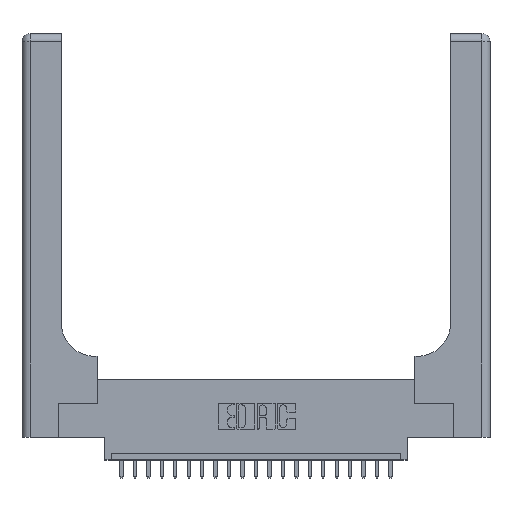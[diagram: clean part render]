
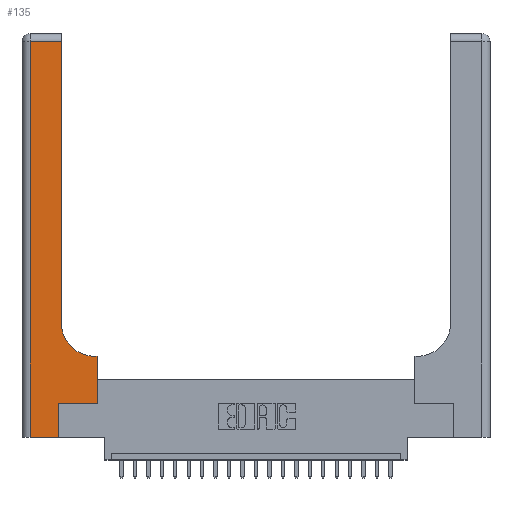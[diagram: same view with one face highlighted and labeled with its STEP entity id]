
A CAD part, top view. The second image highlights one B-rep face of the part: STEP entity #135.
In plain terms, the highlighted planar face has unit normal (0, 0, 1).
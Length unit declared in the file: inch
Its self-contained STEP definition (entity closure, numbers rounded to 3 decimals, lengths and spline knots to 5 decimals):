
#114 = DIRECTION ( 'NONE',  ( 0., 1., 0. ) ) ;
#135 = ADVANCED_FACE ( 'NONE', ( #22724 ), #13976, .F. ) ;
#378 = CARTESIAN_POINT ( 'NONE',  ( 0., 2.94, 0.37 ) ) ;
#489 = VERTEX_POINT ( 'NONE', #5248 ) ;
#940 = CARTESIAN_POINT ( 'NONE',  ( 0., 0., 0.37 ) ) ;
#1065 = CARTESIAN_POINT ( 'NONE',  ( 0.06, 0., 0.37 ) ) ;
#1254 = ORIENTED_EDGE ( 'NONE', *, *, #21619, .T. ) ;
#1466 = DIRECTION ( 'NONE',  ( 0., -1., 0. ) ) ;
#1485 = DIRECTION ( 'NONE',  ( 0., 0., -1. ) ) ;
#1964 = CARTESIAN_POINT ( 'NONE',  ( 0.06, 2.94, 0.37 ) ) ;
#2144 = VERTEX_POINT ( 'NONE', #1065 ) ;
#2228 = CARTESIAN_POINT ( 'NONE',  ( 0.2915, 0.85, 0.37 ) ) ;
#2350 = VERTEX_POINT ( 'NONE', #19064 ) ;
#2406 = VECTOR ( 'NONE', #114, 39.37008 ) ;
#2436 = DIRECTION ( 'NONE',  ( 1., 0., 0. ) ) ;
#3029 = ORIENTED_EDGE ( 'NONE', *, *, #9383, .T. ) ;
#3120 = DIRECTION ( 'NONE',  ( 0., 1., 0. ) ) ;
#3335 = CARTESIAN_POINT ( 'NONE',  ( 0.5585, 0.25, 0.37 ) ) ;
#3462 = DIRECTION ( 'NONE',  ( 1., 0., 0. ) ) ;
#3573 = VERTEX_POINT ( 'NONE', #10100 ) ;
#3940 = EDGE_CURVE ( 'NONE', #23314, #2350, #17801, .T. ) ;
#5221 = VECTOR ( 'NONE', #14301, 39.37008 ) ;
#5248 = CARTESIAN_POINT ( 'NONE',  ( 0.269, 0., 0.37 ) ) ;
#6643 = ORIENTED_EDGE ( 'NONE', *, *, #7763, .T. ) ;
#6750 = VERTEX_POINT ( 'NONE', #1964 ) ;
#7763 = EDGE_CURVE ( 'NONE', #6750, #2144, #15623, .T. ) ;
#8022 = CIRCLE ( 'NONE', #17472, 0.25 ) ;
#8396 = DIRECTION ( 'NONE',  ( 1., 0., 0. ) ) ;
#8469 = VECTOR ( 'NONE', #9694, 39.37008 ) ;
#8691 = CARTESIAN_POINT ( 'NONE',  ( 0.269, 0.25, 0.37 ) ) ;
#8767 = CARTESIAN_POINT ( 'NONE',  ( 0.2915, 3., 0.37 ) ) ;
#8817 = EDGE_LOOP ( 'NONE', ( #12854, #9154, #6643, #3029, #10839, #1254, #19373, #16457, #23929 ) ) ;
#8840 = LINE ( 'NONE', #8767, #20716 ) ;
#8846 = DIRECTION ( 'NONE',  ( 0., 1., 0. ) ) ;
#9154 = ORIENTED_EDGE ( 'NONE', *, *, #10484, .T. ) ;
#9383 = EDGE_CURVE ( 'NONE', #2144, #489, #22143, .T. ) ;
#9637 = CARTESIAN_POINT ( 'NONE',  ( 0.269, 0.25, 0.37 ) ) ;
#9694 = DIRECTION ( 'NONE',  ( -1., 0., 0. ) ) ;
#10100 = CARTESIAN_POINT ( 'NONE',  ( 0.2915, 2.94, 0.37 ) ) ;
#10171 = LINE ( 'NONE', #18533, #5221 ) ;
#10422 = VERTEX_POINT ( 'NONE', #8691 ) ;
#10484 = EDGE_CURVE ( 'NONE', #3573, #6750, #21208, .T. ) ;
#10530 = CARTESIAN_POINT ( 'NONE',  ( 0.5415, 0.6, 0.37 ) ) ;
#10682 = VERTEX_POINT ( 'NONE', #2228 ) ;
#10839 = ORIENTED_EDGE ( 'NONE', *, *, #12359, .T. ) ;
#12359 = EDGE_CURVE ( 'NONE', #489, #10422, #13602, .T. ) ;
#12829 = AXIS2_PLACEMENT_3D ( 'NONE', #23503, #1485, #14568 ) ;
#12854 = ORIENTED_EDGE ( 'NONE', *, *, #23221, .T. ) ;
#13602 = LINE ( 'NONE', #17968, #19414 ) ;
#13976 = PLANE ( 'NONE',  #12829 ) ;
#14301 = DIRECTION ( 'NONE',  ( -1., 0., 0. ) ) ;
#14367 = CARTESIAN_POINT ( 'NONE',  ( 0.06, 3., 0.37 ) ) ;
#14568 = DIRECTION ( 'NONE',  ( -1., 0., 0. ) ) ;
#14589 = CARTESIAN_POINT ( 'NONE',  ( 0.5415, 0.85, 0.37 ) ) ;
#14875 = VERTEX_POINT ( 'NONE', #10530 ) ;
#15623 = LINE ( 'NONE', #14367, #17373 ) ;
#15749 = EDGE_CURVE ( 'NONE', #2350, #14875, #10171, .T. ) ;
#16072 = VECTOR ( 'NONE', #8396, 39.37008 ) ;
#16457 = ORIENTED_EDGE ( 'NONE', *, *, #15749, .T. ) ;
#16778 = CARTESIAN_POINT ( 'NONE',  ( 0.5585, 0.25, 0.37 ) ) ;
#16853 = EDGE_CURVE ( 'NONE', #14875, #10682, #8022, .T. ) ;
#17373 = VECTOR ( 'NONE', #1466, 39.37008 ) ;
#17472 = AXIS2_PLACEMENT_3D ( 'NONE', #14589, #21841, #3462 ) ;
#17801 = LINE ( 'NONE', #16778, #2406 ) ;
#17968 = CARTESIAN_POINT ( 'NONE',  ( 0.269, 0., 0.37 ) ) ;
#18533 = CARTESIAN_POINT ( 'NONE',  ( 0.2915, 0.6, 0.37 ) ) ;
#19064 = CARTESIAN_POINT ( 'NONE',  ( 0.5585, 0.6, 0.37 ) ) ;
#19373 = ORIENTED_EDGE ( 'NONE', *, *, #3940, .T. ) ;
#19414 = VECTOR ( 'NONE', #3120, 39.37008 ) ;
#19417 = LINE ( 'NONE', #9637, #23132 ) ;
#20716 = VECTOR ( 'NONE', #8846, 39.37008 ) ;
#21208 = LINE ( 'NONE', #378, #8469 ) ;
#21619 = EDGE_CURVE ( 'NONE', #10422, #23314, #19417, .T. ) ;
#21841 = DIRECTION ( 'NONE',  ( 0., 0., -1. ) ) ;
#22143 = LINE ( 'NONE', #940, #16072 ) ;
#22724 = FACE_OUTER_BOUND ( 'NONE', #8817, .T. ) ;
#23132 = VECTOR ( 'NONE', #2436, 39.37008 ) ;
#23221 = EDGE_CURVE ( 'NONE', #10682, #3573, #8840, .T. ) ;
#23314 = VERTEX_POINT ( 'NONE', #3335 ) ;
#23503 = CARTESIAN_POINT ( 'NONE',  ( 0., 3., 0.37 ) ) ;
#23929 = ORIENTED_EDGE ( 'NONE', *, *, #16853, .T. ) ;
